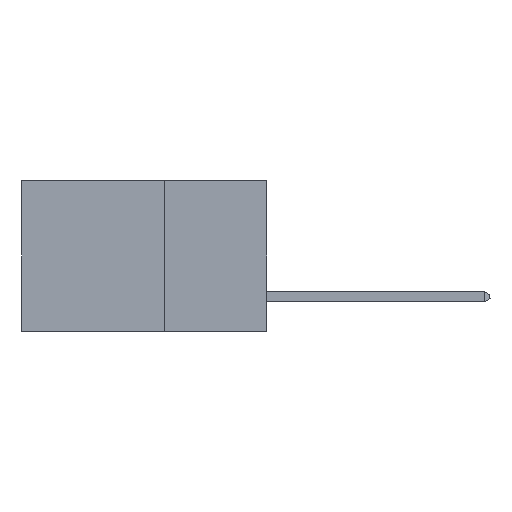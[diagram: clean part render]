
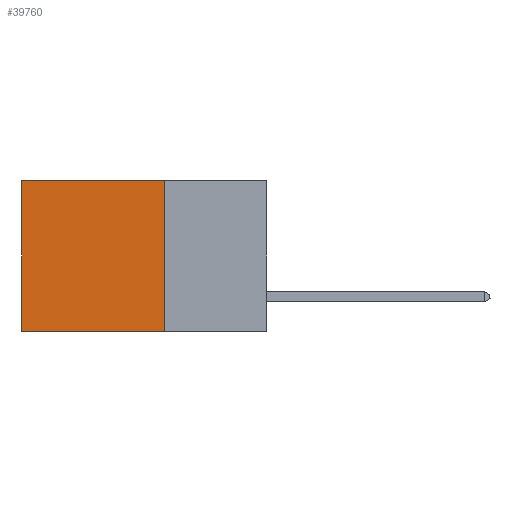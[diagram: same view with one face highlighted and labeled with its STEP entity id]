
A CAD part, left-side view. The second image highlights one B-rep face of the part: STEP entity #39760.
In plain terms, the highlighted planar face has unit normal (-1, 0, 0).
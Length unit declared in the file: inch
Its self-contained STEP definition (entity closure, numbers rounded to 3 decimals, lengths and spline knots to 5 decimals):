
#314 = AXIS2_PLACEMENT_3D ( 'NONE', #43540, #32969, #47275 ) ;
#440 = VERTEX_POINT ( 'NONE', #31562 ) ;
#848 = VERTEX_POINT ( 'NONE', #38327 ) ;
#5116 = ORIENTED_EDGE ( 'NONE', *, *, #39793, .T. ) ;
#6373 = LINE ( 'NONE', #41955, #25347 ) ;
#8294 = ORIENTED_EDGE ( 'NONE', *, *, #31530, .F. ) ;
#8814 = ORIENTED_EDGE ( 'NONE', *, *, #25335, .F. ) ;
#10579 = CARTESIAN_POINT ( 'NONE',  ( 0.2875, 0.25, 0. ) ) ;
#15696 = VECTOR ( 'NONE', #41072, 39.37008 ) ;
#15701 = FACE_OUTER_BOUND ( 'NONE', #47498, .T. ) ;
#18464 = DIRECTION ( 'NONE',  ( 0., 1., 0. ) ) ;
#19247 = DIRECTION ( 'NONE',  ( 0., 0., -1. ) ) ;
#23771 = EDGE_CURVE ( 'NONE', #440, #41326, #6373, .T. ) ;
#24011 = ORIENTED_EDGE ( 'NONE', *, *, #23771, .T. ) ;
#25335 = EDGE_CURVE ( 'NONE', #39562, #41326, #46222, .T. ) ;
#25347 = VECTOR ( 'NONE', #45480, 39.37008 ) ;
#26829 = CARTESIAN_POINT ( 'NONE',  ( 0.2875, 0.25, 0. ) ) ;
#27356 = CARTESIAN_POINT ( 'NONE',  ( 0.2875, 0.25, -0.37 ) ) ;
#30713 = LINE ( 'NONE', #10579, #47344 ) ;
#31530 = EDGE_CURVE ( 'NONE', #848, #39562, #44577, .T. ) ;
#31562 = CARTESIAN_POINT ( 'NONE',  ( 0.2875, 0.6, 0. ) ) ;
#32969 = DIRECTION ( 'NONE',  ( 1., 0., 0. ) ) ;
#34204 = CARTESIAN_POINT ( 'NONE',  ( 0.2875, 0.25, -0.37 ) ) ;
#35671 = CARTESIAN_POINT ( 'NONE',  ( 0.2875, 0.6, -0.37 ) ) ;
#38327 = CARTESIAN_POINT ( 'NONE',  ( 0.2875, 0.25, 0. ) ) ;
#39435 = VECTOR ( 'NONE', #19247, 39.37008 ) ;
#39562 = VERTEX_POINT ( 'NONE', #27356 ) ;
#39760 = ADVANCED_FACE ( 'NONE', ( #15701 ), #47116, .F. ) ;
#39793 = EDGE_CURVE ( 'NONE', #848, #440, #30713, .T. ) ;
#41072 = DIRECTION ( 'NONE',  ( 0., 1., 0. ) ) ;
#41326 = VERTEX_POINT ( 'NONE', #35671 ) ;
#41955 = CARTESIAN_POINT ( 'NONE',  ( 0.2875, 0.6, 0. ) ) ;
#43540 = CARTESIAN_POINT ( 'NONE',  ( 0.2875, 0.25, 0. ) ) ;
#44577 = LINE ( 'NONE', #26829, #39435 ) ;
#45480 = DIRECTION ( 'NONE',  ( 0., 0., -1. ) ) ;
#46222 = LINE ( 'NONE', #34204, #15696 ) ;
#47116 = PLANE ( 'NONE',  #314 ) ;
#47275 = DIRECTION ( 'NONE',  ( 0., 0., -1. ) ) ;
#47344 = VECTOR ( 'NONE', #18464, 39.37008 ) ;
#47498 = EDGE_LOOP ( 'NONE', ( #24011, #8814, #8294, #5116 ) ) ;
